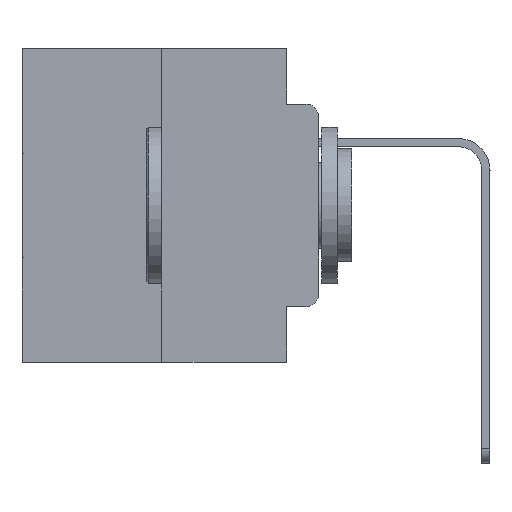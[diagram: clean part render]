
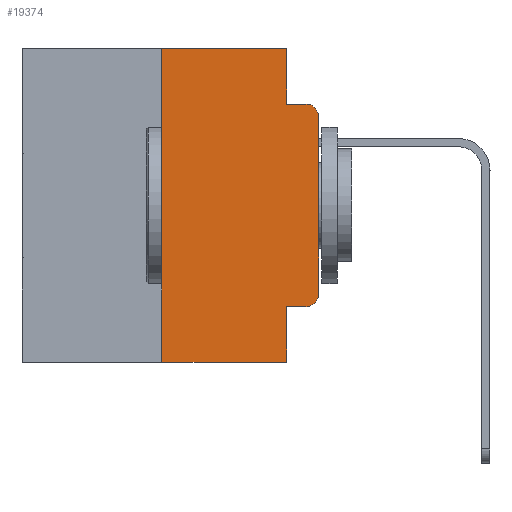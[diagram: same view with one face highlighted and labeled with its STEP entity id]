
A CAD part, left-side view. The second image highlights one B-rep face of the part: STEP entity #19374.
In plain terms, the highlighted planar face has unit normal (-1, 0, 0).
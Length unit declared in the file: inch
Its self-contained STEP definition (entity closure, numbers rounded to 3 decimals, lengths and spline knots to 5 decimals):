
#111 = CARTESIAN_POINT ( 'NONE',  ( 0., 0.051, -0.4115 ) ) ;
#204 = DIRECTION ( 'NONE',  ( 0., -1., 0. ) ) ;
#283 = LINE ( 'NONE', #111, #5213 ) ;
#456 = FACE_OUTER_BOUND ( 'NONE', #2038, .T. ) ;
#503 = VECTOR ( 'NONE', #12716, 39.37008 ) ;
#578 = ORIENTED_EDGE ( 'NONE', *, *, #22882, .T. ) ;
#1298 = LINE ( 'NONE', #14943, #24460 ) ;
#1304 = CARTESIAN_POINT ( 'NONE',  ( 0., 0.473, 0. ) ) ;
#1467 = DIRECTION ( 'NONE',  ( 0., 0., -1. ) ) ;
#1616 = VECTOR ( 'NONE', #19903, 39.37008 ) ;
#1709 = DIRECTION ( 'NONE',  ( 0., 0., 1. ) ) ;
#2038 = EDGE_LOOP ( 'NONE', ( #20587, #23825, #20991, #13827, #16555, #17739, #578, #11165, #3049, #9029 ) ) ;
#2327 = VERTEX_POINT ( 'NONE', #11389 ) ;
#2841 = DIRECTION ( 'NONE',  ( 0., -1., 0. ) ) ;
#3038 = EDGE_CURVE ( 'NONE', #2327, #16913, #7627, .T. ) ;
#3049 = ORIENTED_EDGE ( 'NONE', *, *, #22245, .T. ) ;
#3874 = CARTESIAN_POINT ( 'NONE',  ( 0., 0., -0.1085 ) ) ;
#4067 = DIRECTION ( 'NONE',  ( 0., 0., -1. ) ) ;
#4657 = CARTESIAN_POINT ( 'NONE',  ( 0., 0.02, -0.1085 ) ) ;
#4873 = VECTOR ( 'NONE', #1709, 39.37008 ) ;
#5213 = VECTOR ( 'NONE', #204, 39.37008 ) ;
#5371 = DIRECTION ( 'NONE',  ( 0., 0., -1. ) ) ;
#5426 = VECTOR ( 'NONE', #4067, 39.37008 ) ;
#5466 = PLANE ( 'NONE',  #16795 ) ;
#5539 = VERTEX_POINT ( 'NONE', #16691 ) ;
#5893 = CARTESIAN_POINT ( 'NONE',  ( 0., 0., -0.3915 ) ) ;
#6354 = CIRCLE ( 'NONE', #25225, 0.02 ) ;
#6883 = AXIS2_PLACEMENT_3D ( 'NONE', #4657, #20208, #16129 ) ;
#7283 = VERTEX_POINT ( 'NONE', #5893 ) ;
#7627 = LINE ( 'NONE', #11051, #1616 ) ;
#8203 = EDGE_CURVE ( 'NONE', #14590, #11549, #9478, .T. ) ;
#9029 = ORIENTED_EDGE ( 'NONE', *, *, #10192, .T. ) ;
#9478 = LINE ( 'NONE', #24454, #4873 ) ;
#10160 = VERTEX_POINT ( 'NONE', #3874 ) ;
#10192 = EDGE_CURVE ( 'NONE', #18142, #7283, #6354, .T. ) ;
#11051 = CARTESIAN_POINT ( 'NONE',  ( 0., 0.051, -0.0885 ) ) ;
#11165 = ORIENTED_EDGE ( 'NONE', *, *, #22550, .F. ) ;
#11389 = CARTESIAN_POINT ( 'NONE',  ( 0., 0.051, -0.0885 ) ) ;
#11549 = VERTEX_POINT ( 'NONE', #18107 ) ;
#12061 = EDGE_CURVE ( 'NONE', #10160, #16913, #24774, .T. ) ;
#12716 = DIRECTION ( 'NONE',  ( 0., -1., 0. ) ) ;
#13016 = CARTESIAN_POINT ( 'NONE',  ( 0., 0.051, 0. ) ) ;
#13827 = ORIENTED_EDGE ( 'NONE', *, *, #19601, .F. ) ;
#13898 = CARTESIAN_POINT ( 'NONE',  ( 0., 0.25, -0.5 ) ) ;
#14170 = VECTOR ( 'NONE', #23089, 39.37008 ) ;
#14303 = DIRECTION ( 'NONE',  ( 1., 0., 0. ) ) ;
#14590 = VERTEX_POINT ( 'NONE', #13898 ) ;
#14598 = CARTESIAN_POINT ( 'NONE',  ( 0., 0.051, -0.5 ) ) ;
#14943 = CARTESIAN_POINT ( 'NONE',  ( 0., 0.051, 0. ) ) ;
#16129 = DIRECTION ( 'NONE',  ( 0., 0., -1. ) ) ;
#16426 = VECTOR ( 'NONE', #2841, 39.37008 ) ;
#16555 = ORIENTED_EDGE ( 'NONE', *, *, #23807, .F. ) ;
#16656 = LINE ( 'NONE', #13016, #5426 ) ;
#16691 = CARTESIAN_POINT ( 'NONE',  ( 0., 0.051, 0. ) ) ;
#16795 = AXIS2_PLACEMENT_3D ( 'NONE', #23375, #14303, #5371 ) ;
#16896 = EDGE_CURVE ( 'NONE', #7283, #10160, #20083, .T. ) ;
#16913 = VERTEX_POINT ( 'NONE', #27794 ) ;
#17694 = DIRECTION ( 'NONE',  ( -1., 0., 0. ) ) ;
#17739 = ORIENTED_EDGE ( 'NONE', *, *, #8203, .F. ) ;
#18107 = CARTESIAN_POINT ( 'NONE',  ( 0., 0.25, 0. ) ) ;
#18142 = VERTEX_POINT ( 'NONE', #18987 ) ;
#18581 = CARTESIAN_POINT ( 'NONE',  ( 0., 0., 0. ) ) ;
#18987 = CARTESIAN_POINT ( 'NONE',  ( 0., 0.02, -0.4115 ) ) ;
#19374 = ADVANCED_FACE ( 'NONE', ( #456 ), #5466, .F. ) ;
#19601 = EDGE_CURVE ( 'NONE', #5539, #2327, #16656, .T. ) ;
#19903 = DIRECTION ( 'NONE',  ( 0., -1., 0. ) ) ;
#20083 = LINE ( 'NONE', #18581, #14170 ) ;
#20121 = CARTESIAN_POINT ( 'NONE',  ( 0., 0.02, -0.3915 ) ) ;
#20208 = DIRECTION ( 'NONE',  ( -1., 0., 0. ) ) ;
#20587 = ORIENTED_EDGE ( 'NONE', *, *, #16896, .T. ) ;
#20991 = ORIENTED_EDGE ( 'NONE', *, *, #3038, .F. ) ;
#21691 = CARTESIAN_POINT ( 'NONE',  ( 0., 0.051, -0.4115 ) ) ;
#22245 = EDGE_CURVE ( 'NONE', #27729, #18142, #283, .T. ) ;
#22550 = EDGE_CURVE ( 'NONE', #27729, #27049, #1298, .T. ) ;
#22882 = EDGE_CURVE ( 'NONE', #14590, #27049, #26549, .T. ) ;
#23089 = DIRECTION ( 'NONE',  ( 0., 0., 1. ) ) ;
#23375 = CARTESIAN_POINT ( 'NONE',  ( 0., 0.473, 0. ) ) ;
#23807 = EDGE_CURVE ( 'NONE', #11549, #5539, #27895, .T. ) ;
#23825 = ORIENTED_EDGE ( 'NONE', *, *, #12061, .T. ) ;
#24454 = CARTESIAN_POINT ( 'NONE',  ( 0., 0.25, 0. ) ) ;
#24460 = VECTOR ( 'NONE', #1467, 39.37008 ) ;
#24774 = CIRCLE ( 'NONE', #6883, 0.02 ) ;
#25225 = AXIS2_PLACEMENT_3D ( 'NONE', #20121, #17694, #26705 ) ;
#26549 = LINE ( 'NONE', #27448, #16426 ) ;
#26705 = DIRECTION ( 'NONE',  ( 0., 0., -1. ) ) ;
#27049 = VERTEX_POINT ( 'NONE', #14598 ) ;
#27448 = CARTESIAN_POINT ( 'NONE',  ( 0., 0.473, -0.5 ) ) ;
#27729 = VERTEX_POINT ( 'NONE', #21691 ) ;
#27794 = CARTESIAN_POINT ( 'NONE',  ( 0., 0.02, -0.0885 ) ) ;
#27895 = LINE ( 'NONE', #1304, #503 ) ;
